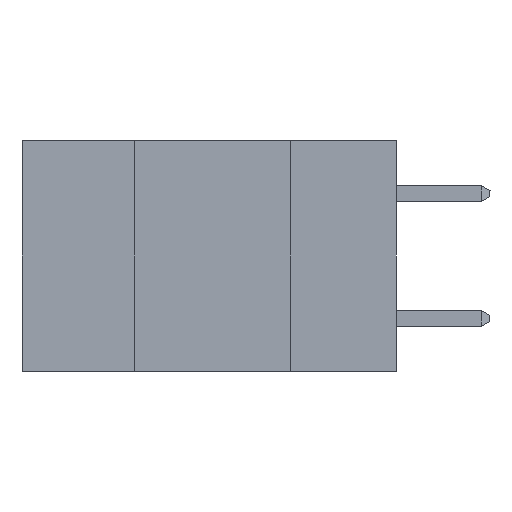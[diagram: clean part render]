
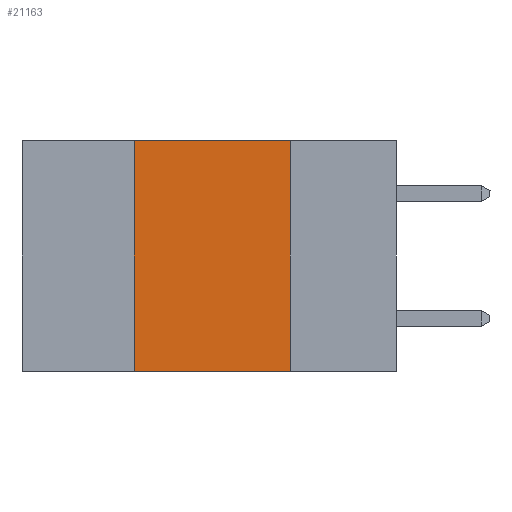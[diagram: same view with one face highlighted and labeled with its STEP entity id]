
A CAD part, left-side view. The second image highlights one B-rep face of the part: STEP entity #21163.
In plain terms, the highlighted planar face has unit normal (-1, 0, 0).
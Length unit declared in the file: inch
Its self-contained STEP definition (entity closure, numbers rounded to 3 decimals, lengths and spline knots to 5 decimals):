
#365 = LINE ( 'NONE', #20101, #32245 ) ;
#1005 = CARTESIAN_POINT ( 'NONE',  ( 0., 0.6, 0. ) ) ;
#1790 = AXIS2_PLACEMENT_3D ( 'NONE', #21157, #5694, #23810 ) ;
#3596 = DIRECTION ( 'NONE',  ( 0., -1., 0. ) ) ;
#3908 = VERTEX_POINT ( 'NONE', #31921 ) ;
#3961 = VERTEX_POINT ( 'NONE', #17577 ) ;
#4305 = ORIENTED_EDGE ( 'NONE', *, *, #10207, .F. ) ;
#4782 = VECTOR ( 'NONE', #23217, 39.37008 ) ;
#5694 = DIRECTION ( 'NONE',  ( 1., 0., 0. ) ) ;
#5811 = CARTESIAN_POINT ( 'NONE',  ( 0., 0.17, -0.37 ) ) ;
#7398 = DIRECTION ( 'NONE',  ( 0., 0., -1. ) ) ;
#7543 = VECTOR ( 'NONE', #3596, 39.37008 ) ;
#7617 = ORIENTED_EDGE ( 'NONE', *, *, #30802, .T. ) ;
#9964 = DIRECTION ( 'NONE',  ( 0., 0., 1. ) ) ;
#10207 = EDGE_CURVE ( 'NONE', #3908, #30287, #365, .T. ) ;
#11604 = EDGE_CURVE ( 'NONE', #3961, #13027, #29551, .T. ) ;
#13027 = VERTEX_POINT ( 'NONE', #27131 ) ;
#14179 = FACE_OUTER_BOUND ( 'NONE', #15861, .T. ) ;
#15861 = EDGE_LOOP ( 'NONE', ( #4305, #26483, #25863, #7617 ) ) ;
#15955 = PLANE ( 'NONE',  #1790 ) ;
#17577 = CARTESIAN_POINT ( 'NONE',  ( 0., 0.42, -0.37 ) ) ;
#20101 = CARTESIAN_POINT ( 'NONE',  ( 0., 0.17, 0. ) ) ;
#20527 = CARTESIAN_POINT ( 'NONE',  ( 0., 0.6, -0.37 ) ) ;
#21157 = CARTESIAN_POINT ( 'NONE',  ( 0., 0.6, 0. ) ) ;
#21163 = ADVANCED_FACE ( 'NONE', ( #14179 ), #15955, .F. ) ;
#22688 = VECTOR ( 'NONE', #9964, 39.37008 ) ;
#23217 = DIRECTION ( 'NONE',  ( 0., -1., 0. ) ) ;
#23810 = DIRECTION ( 'NONE',  ( 0., 0., -1. ) ) ;
#25863 = ORIENTED_EDGE ( 'NONE', *, *, #11604, .F. ) ;
#26483 = ORIENTED_EDGE ( 'NONE', *, *, #31776, .F. ) ;
#27131 = CARTESIAN_POINT ( 'NONE',  ( 0., 0.42, 0. ) ) ;
#27941 = CARTESIAN_POINT ( 'NONE',  ( 0., 0.42, 0. ) ) ;
#28209 = LINE ( 'NONE', #1005, #7543 ) ;
#29551 = LINE ( 'NONE', #27941, #22688 ) ;
#30287 = VERTEX_POINT ( 'NONE', #5811 ) ;
#30802 = EDGE_CURVE ( 'NONE', #3961, #30287, #32230, .T. ) ;
#31776 = EDGE_CURVE ( 'NONE', #13027, #3908, #28209, .T. ) ;
#31921 = CARTESIAN_POINT ( 'NONE',  ( 0., 0.17, 0. ) ) ;
#32230 = LINE ( 'NONE', #20527, #4782 ) ;
#32245 = VECTOR ( 'NONE', #7398, 39.37008 ) ;
